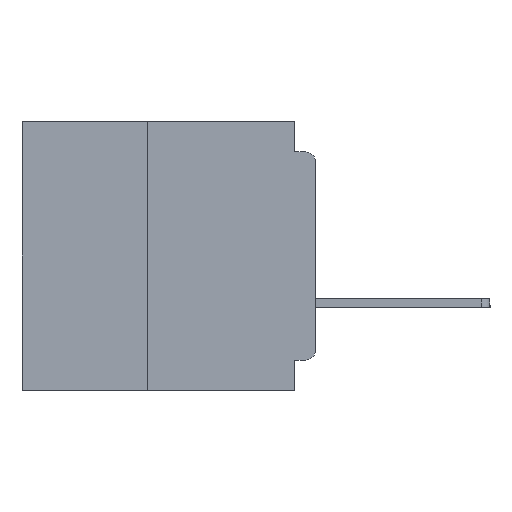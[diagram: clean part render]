
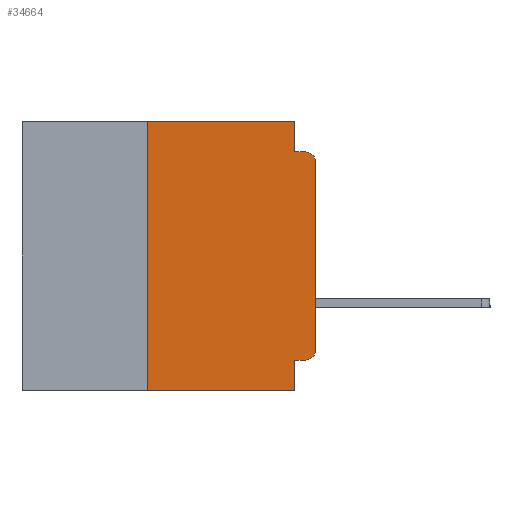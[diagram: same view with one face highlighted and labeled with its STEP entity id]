
A CAD part, left-side view. The second image highlights one B-rep face of the part: STEP entity #34664.
In plain terms, the highlighted planar face has unit normal (-1, 0, 0).
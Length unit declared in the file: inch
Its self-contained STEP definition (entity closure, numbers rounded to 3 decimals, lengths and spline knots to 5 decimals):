
#1065 = EDGE_CURVE ( 'NONE', #49664, #34833, #6896, .T. ) ;
#1662 = LINE ( 'NONE', #41912, #49537 ) ;
#3063 = CARTESIAN_POINT ( 'NONE',  ( 0., 0., -0.06 ) ) ;
#3783 = EDGE_CURVE ( 'NONE', #22561, #9549, #44619, .T. ) ;
#4071 = EDGE_CURVE ( 'NONE', #33693, #4332, #31582, .T. ) ;
#4259 = CARTESIAN_POINT ( 'NONE',  ( 0., 0.015, -0.045 ) ) ;
#4280 = ORIENTED_EDGE ( 'NONE', *, *, #49080, .F. ) ;
#4332 = VERTEX_POINT ( 'NONE', #4259 ) ;
#6644 = CARTESIAN_POINT ( 'NONE',  ( 0., 0.031, -0.355 ) ) ;
#6896 = LINE ( 'NONE', #49547, #42390 ) ;
#7435 = VECTOR ( 'NONE', #31156, 39.37008 ) ;
#9538 = DIRECTION ( 'NONE',  ( 0., -1., 0. ) ) ;
#9549 = VERTEX_POINT ( 'NONE', #13468 ) ;
#10004 = ORIENTED_EDGE ( 'NONE', *, *, #34157, .F. ) ;
#10330 = PLANE ( 'NONE',  #44743 ) ;
#11447 = CARTESIAN_POINT ( 'NONE',  ( 0., 0.015, -0.06 ) ) ;
#12524 = VERTEX_POINT ( 'NONE', #31113 ) ;
#13468 = CARTESIAN_POINT ( 'NONE',  ( 0., 0.031, -0.4 ) ) ;
#14981 = DIRECTION ( 'NONE',  ( 1., 0., 0. ) ) ;
#15448 = ORIENTED_EDGE ( 'NONE', *, *, #30579, .F. ) ;
#15883 = CARTESIAN_POINT ( 'NONE',  ( 0., 0.25, 0. ) ) ;
#16077 = DIRECTION ( 'NONE',  ( 0., 0., -1. ) ) ;
#17622 = DIRECTION ( 'NONE',  ( -1., 0., 0. ) ) ;
#17731 = CARTESIAN_POINT ( 'NONE',  ( 0., 0.437, -0.4 ) ) ;
#18617 = AXIS2_PLACEMENT_3D ( 'NONE', #11447, #43803, #16077 ) ;
#19063 = LINE ( 'NONE', #48266, #42194 ) ;
#21277 = LINE ( 'NONE', #58823, #7435 ) ;
#21560 = DIRECTION ( 'NONE',  ( 0., 0., -1. ) ) ;
#22213 = DIRECTION ( 'NONE',  ( 0., -1., 0. ) ) ;
#22334 = VECTOR ( 'NONE', #21560, 39.37008 ) ;
#22426 = ORIENTED_EDGE ( 'NONE', *, *, #22831, .F. ) ;
#22561 = VERTEX_POINT ( 'NONE', #47267 ) ;
#22831 = EDGE_CURVE ( 'NONE', #23317, #9549, #34590, .T. ) ;
#22999 = VERTEX_POINT ( 'NONE', #46016 ) ;
#23317 = VERTEX_POINT ( 'NONE', #6644 ) ;
#26044 = CARTESIAN_POINT ( 'NONE',  ( 0., 0.031, -0.4 ) ) ;
#26331 = ORIENTED_EDGE ( 'NONE', *, *, #1065, .F. ) ;
#26731 = DIRECTION ( 'NONE',  ( 0., -1., 0. ) ) ;
#28482 = FACE_OUTER_BOUND ( 'NONE', #32610, .T. ) ;
#30051 = AXIS2_PLACEMENT_3D ( 'NONE', #45358, #17622, #50005 ) ;
#30579 = EDGE_CURVE ( 'NONE', #53609, #23317, #37861, .T. ) ;
#31113 = CARTESIAN_POINT ( 'NONE',  ( 0., 0., -0.34 ) ) ;
#31156 = DIRECTION ( 'NONE',  ( 0., 0., 1. ) ) ;
#31582 = CIRCLE ( 'NONE', #18617, 0.015 ) ;
#32610 = EDGE_LOOP ( 'NONE', ( #34353, #42287, #57929, #10004, #26331, #4280, #35125, #22426, #15448, #57571 ) ) ;
#33693 = VERTEX_POINT ( 'NONE', #3063 ) ;
#34157 = EDGE_CURVE ( 'NONE', #34833, #22999, #19063, .T. ) ;
#34353 = ORIENTED_EDGE ( 'NONE', *, *, #51655, .T. ) ;
#34553 = DIRECTION ( 'NONE',  ( 0., 0., 1. ) ) ;
#34590 = LINE ( 'NONE', #26044, #22334 ) ;
#34664 = ADVANCED_FACE ( 'NONE', ( #28482 ), #10330, .F. ) ;
#34833 = VERTEX_POINT ( 'NONE', #53407 ) ;
#35125 = ORIENTED_EDGE ( 'NONE', *, *, #3783, .T. ) ;
#36423 = VECTOR ( 'NONE', #41001, 39.37008 ) ;
#37697 = CIRCLE ( 'NONE', #30051, 0.015 ) ;
#37861 = LINE ( 'NONE', #54756, #36423 ) ;
#39112 = DIRECTION ( 'NONE',  ( 0., 0., -1. ) ) ;
#41001 = DIRECTION ( 'NONE',  ( 0., 1., 0. ) ) ;
#41912 = CARTESIAN_POINT ( 'NONE',  ( 0., 0., -0.045 ) ) ;
#42194 = VECTOR ( 'NONE', #39112, 39.37008 ) ;
#42287 = ORIENTED_EDGE ( 'NONE', *, *, #4071, .T. ) ;
#42390 = VECTOR ( 'NONE', #26731, 39.37008 ) ;
#43803 = DIRECTION ( 'NONE',  ( -1., 0., 0. ) ) ;
#44364 = LINE ( 'NONE', #57629, #56640 ) ;
#44619 = LINE ( 'NONE', #17731, #55454 ) ;
#44743 = AXIS2_PLACEMENT_3D ( 'NONE', #51804, #14981, #47388 ) ;
#45269 = CARTESIAN_POINT ( 'NONE',  ( 0., 0.015, -0.355 ) ) ;
#45358 = CARTESIAN_POINT ( 'NONE',  ( 0., 0.015, -0.34 ) ) ;
#46016 = CARTESIAN_POINT ( 'NONE',  ( 0., 0.031, -0.045 ) ) ;
#47267 = CARTESIAN_POINT ( 'NONE',  ( 0., 0.25, -0.4 ) ) ;
#47388 = DIRECTION ( 'NONE',  ( 0., 0., -1. ) ) ;
#48266 = CARTESIAN_POINT ( 'NONE',  ( 0., 0.031, 0. ) ) ;
#48310 = EDGE_CURVE ( 'NONE', #22999, #4332, #1662, .T. ) ;
#49080 = EDGE_CURVE ( 'NONE', #22561, #49664, #44364, .T. ) ;
#49537 = VECTOR ( 'NONE', #9538, 39.37008 ) ;
#49547 = CARTESIAN_POINT ( 'NONE',  ( 0., 0.437, 0. ) ) ;
#49664 = VERTEX_POINT ( 'NONE', #15883 ) ;
#50005 = DIRECTION ( 'NONE',  ( 0., 0., -1. ) ) ;
#51655 = EDGE_CURVE ( 'NONE', #12524, #33693, #21277, .T. ) ;
#51804 = CARTESIAN_POINT ( 'NONE',  ( 0., 0.437, 0. ) ) ;
#53407 = CARTESIAN_POINT ( 'NONE',  ( 0., 0.031, 0. ) ) ;
#53609 = VERTEX_POINT ( 'NONE', #45269 ) ;
#54756 = CARTESIAN_POINT ( 'NONE',  ( 0., 0., -0.355 ) ) ;
#55454 = VECTOR ( 'NONE', #22213, 39.37008 ) ;
#56640 = VECTOR ( 'NONE', #34553, 39.37008 ) ;
#56751 = EDGE_CURVE ( 'NONE', #53609, #12524, #37697, .T. ) ;
#57571 = ORIENTED_EDGE ( 'NONE', *, *, #56751, .T. ) ;
#57629 = CARTESIAN_POINT ( 'NONE',  ( 0., 0.25, -0.4 ) ) ;
#57929 = ORIENTED_EDGE ( 'NONE', *, *, #48310, .F. ) ;
#58823 = CARTESIAN_POINT ( 'NONE',  ( 0., 0., 0. ) ) ;
